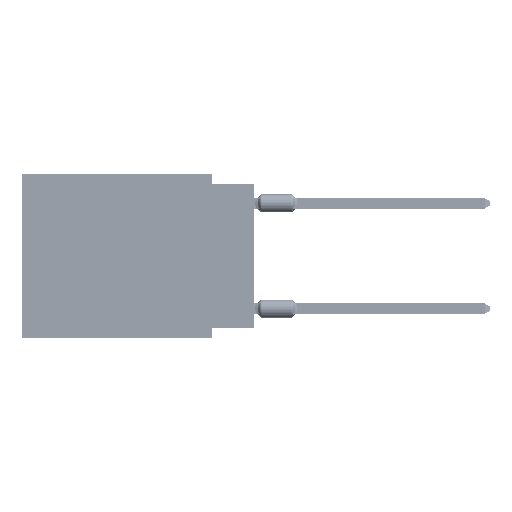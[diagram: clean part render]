
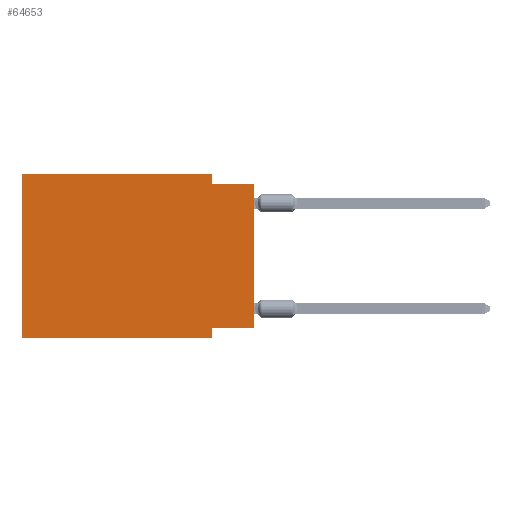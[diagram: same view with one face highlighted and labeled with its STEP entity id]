
A CAD part, left-side view. The second image highlights one B-rep face of the part: STEP entity #64653.
In plain terms, the highlighted planar face has unit normal (-1, 0, 0).
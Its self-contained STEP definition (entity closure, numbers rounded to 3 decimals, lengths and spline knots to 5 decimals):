
#2459 = CARTESIAN_POINT ( 'NONE',  ( 0., 0.1, -0.365 ) ) ;
#3031 = VERTEX_POINT ( 'NONE', #11436 ) ;
#4099 = EDGE_CURVE ( 'NONE', #5840, #3031, #73154, .T. ) ;
#5372 = PLANE ( 'NONE',  #74616 ) ;
#5840 = VERTEX_POINT ( 'NONE', #71254 ) ;
#6449 = CARTESIAN_POINT ( 'NONE',  ( 0., 0., -0.365 ) ) ;
#7087 = ORIENTED_EDGE ( 'NONE', *, *, #54400, .F. ) ;
#7628 = DIRECTION ( 'NONE',  ( 0., 0., 1. ) ) ;
#7770 = CARTESIAN_POINT ( 'NONE',  ( 0., 0.1, -0.39 ) ) ;
#8478 = CARTESIAN_POINT ( 'NONE',  ( 0., 0.1, -0.025 ) ) ;
#9764 = LINE ( 'NONE', #21141, #15468 ) ;
#10652 = DIRECTION ( 'NONE',  ( 1., 0., 0. ) ) ;
#10788 = ORIENTED_EDGE ( 'NONE', *, *, #27793, .T. ) ;
#11131 = ORIENTED_EDGE ( 'NONE', *, *, #4099, .F. ) ;
#11436 = CARTESIAN_POINT ( 'NONE',  ( 0., 0.55, 0. ) ) ;
#12158 = DIRECTION ( 'NONE',  ( 0., -1., 0. ) ) ;
#14091 = LINE ( 'NONE', #69310, #32177 ) ;
#15354 = ORIENTED_EDGE ( 'NONE', *, *, #17006, .F. ) ;
#15468 = VECTOR ( 'NONE', #70698, 39.37008 ) ;
#17006 = EDGE_CURVE ( 'NONE', #20272, #67050, #50319, .T. ) ;
#17376 = VERTEX_POINT ( 'NONE', #2459 ) ;
#17536 = CARTESIAN_POINT ( 'NONE',  ( 0., 0.55, 0. ) ) ;
#18146 = ORIENTED_EDGE ( 'NONE', *, *, #77141, .F. ) ;
#20183 = LINE ( 'NONE', #6449, #28665 ) ;
#20272 = VERTEX_POINT ( 'NONE', #8478 ) ;
#21141 = CARTESIAN_POINT ( 'NONE',  ( 0., 0.55, 0. ) ) ;
#22209 = VECTOR ( 'NONE', #39620, 39.37008 ) ;
#24926 = VECTOR ( 'NONE', #41483, 39.37008 ) ;
#27139 = EDGE_LOOP ( 'NONE', ( #10788, #15354, #18146, #71452, #11131, #65119, #7087, #56127 ) ) ;
#27793 = EDGE_CURVE ( 'NONE', #43552, #67050, #55979, .T. ) ;
#28665 = VECTOR ( 'NONE', #44553, 39.37008 ) ;
#30565 = VERTEX_POINT ( 'NONE', #41671 ) ;
#32177 = VECTOR ( 'NONE', #32724, 39.37008 ) ;
#32724 = DIRECTION ( 'NONE',  ( 0., -1., 0. ) ) ;
#33637 = EDGE_CURVE ( 'NONE', #43552, #17376, #20183, .T. ) ;
#34460 = VECTOR ( 'NONE', #12158, 39.37008 ) ;
#37823 = CARTESIAN_POINT ( 'NONE',  ( 0., 0.1, 0. ) ) ;
#38897 = CARTESIAN_POINT ( 'NONE',  ( 0., 0., -0.025 ) ) ;
#39620 = DIRECTION ( 'NONE',  ( 0., 0., -1. ) ) ;
#41483 = DIRECTION ( 'NONE',  ( 0., 0., 1. ) ) ;
#41671 = CARTESIAN_POINT ( 'NONE',  ( 0., 0.1, 0. ) ) ;
#43125 = DIRECTION ( 'NONE',  ( 0., 0., -1. ) ) ;
#43552 = VERTEX_POINT ( 'NONE', #78934 ) ;
#44553 = DIRECTION ( 'NONE',  ( 0., 1., 0. ) ) ;
#45708 = LINE ( 'NONE', #70489, #22209 ) ;
#46464 = EDGE_CURVE ( 'NONE', #5840, #59261, #14091, .T. ) ;
#47748 = VECTOR ( 'NONE', #7628, 39.37008 ) ;
#50319 = LINE ( 'NONE', #56025, #34460 ) ;
#51655 = EDGE_CURVE ( 'NONE', #3031, #30565, #9764, .T. ) ;
#54400 = EDGE_CURVE ( 'NONE', #17376, #59261, #45708, .T. ) ;
#54916 = CARTESIAN_POINT ( 'NONE',  ( 0., 0.55, 0. ) ) ;
#55334 = DIRECTION ( 'NONE',  ( 0., 0., -1. ) ) ;
#55979 = LINE ( 'NONE', #69339, #47748 ) ;
#56025 = CARTESIAN_POINT ( 'NONE',  ( 0., 0., -0.025 ) ) ;
#56127 = ORIENTED_EDGE ( 'NONE', *, *, #33637, .F. ) ;
#59261 = VERTEX_POINT ( 'NONE', #7770 ) ;
#61142 = VECTOR ( 'NONE', #43125, 39.37008 ) ;
#61415 = LINE ( 'NONE', #37823, #61142 ) ;
#64653 = ADVANCED_FACE ( 'NONE', ( #66296 ), #5372, .F. ) ;
#65119 = ORIENTED_EDGE ( 'NONE', *, *, #46464, .T. ) ;
#66296 = FACE_OUTER_BOUND ( 'NONE', #27139, .T. ) ;
#67050 = VERTEX_POINT ( 'NONE', #38897 ) ;
#69310 = CARTESIAN_POINT ( 'NONE',  ( 0., 0.55, -0.39 ) ) ;
#69339 = CARTESIAN_POINT ( 'NONE',  ( 0., 0., 0. ) ) ;
#70489 = CARTESIAN_POINT ( 'NONE',  ( 0., 0.1, -0.39 ) ) ;
#70698 = DIRECTION ( 'NONE',  ( 0., -1., 0. ) ) ;
#71254 = CARTESIAN_POINT ( 'NONE',  ( 0., 0.55, -0.39 ) ) ;
#71452 = ORIENTED_EDGE ( 'NONE', *, *, #51655, .F. ) ;
#73154 = LINE ( 'NONE', #17536, #24926 ) ;
#74616 = AXIS2_PLACEMENT_3D ( 'NONE', #54916, #10652, #55334 ) ;
#77141 = EDGE_CURVE ( 'NONE', #30565, #20272, #61415, .T. ) ;
#78934 = CARTESIAN_POINT ( 'NONE',  ( 0., 0., -0.365 ) ) ;
